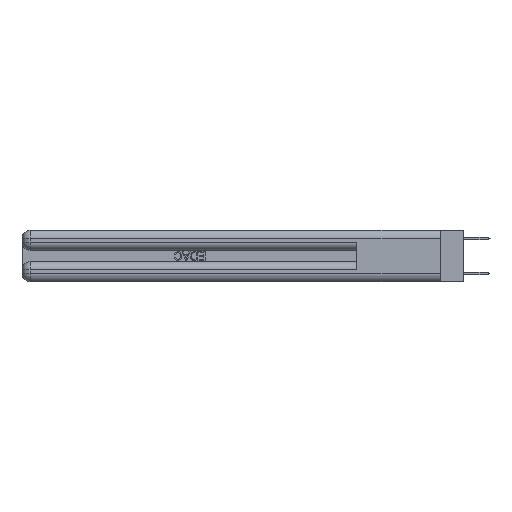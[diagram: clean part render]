
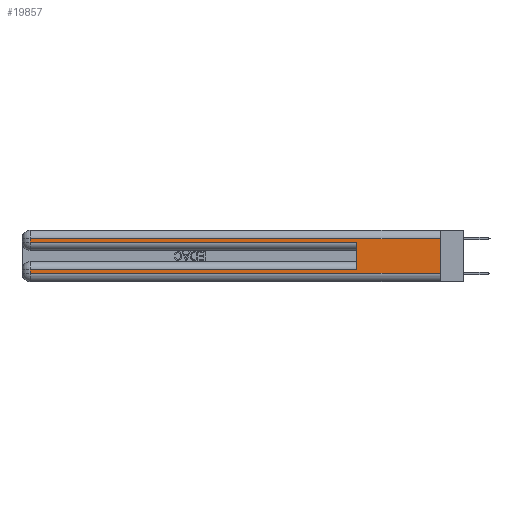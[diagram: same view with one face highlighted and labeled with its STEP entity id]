
A CAD part, left-side view. The second image highlights one B-rep face of the part: STEP entity #19857.
In plain terms, the highlighted planar face has unit normal (-1, 0, 0).
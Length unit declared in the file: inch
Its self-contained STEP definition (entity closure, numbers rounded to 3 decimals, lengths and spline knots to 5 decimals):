
#823 = ORIENTED_EDGE ( 'NONE', *, *, #7670, .T. ) ;
#1004 = CARTESIAN_POINT ( 'NONE',  ( 0., 2.94, 0.085 ) ) ;
#1013 = VECTOR ( 'NONE', #11278, 39.37008 ) ;
#1174 = CARTESIAN_POINT ( 'NONE',  ( 0., 2.94, 0.06 ) ) ;
#1431 = CARTESIAN_POINT ( 'NONE',  ( 0., 0., 0.085 ) ) ;
#1805 = LINE ( 'NONE', #6803, #30430 ) ;
#3520 = LINE ( 'NONE', #14603, #1013 ) ;
#3938 = DIRECTION ( 'NONE',  ( 0., -1., 0. ) ) ;
#4311 = ORIENTED_EDGE ( 'NONE', *, *, #22354, .T. ) ;
#4342 = LINE ( 'NONE', #21496, #29315 ) ;
#4529 = DIRECTION ( 'NONE',  ( 0., 1., 0. ) ) ;
#4663 = ORIENTED_EDGE ( 'NONE', *, *, #34394, .T. ) ;
#5802 = CARTESIAN_POINT ( 'NONE',  ( 0., 0., 0.37 ) ) ;
#6803 = CARTESIAN_POINT ( 'NONE',  ( 0., 0.6, 0.145 ) ) ;
#7670 = EDGE_CURVE ( 'NONE', #19176, #29488, #26688, .T. ) ;
#7906 = CARTESIAN_POINT ( 'NONE',  ( 0., 2.94, 0.37 ) ) ;
#8914 = PLANE ( 'NONE',  #16601 ) ;
#9913 = DIRECTION ( 'NONE',  ( 0., 1., 0. ) ) ;
#10883 = EDGE_CURVE ( 'NONE', #29488, #16420, #21374, .T. ) ;
#11278 = DIRECTION ( 'NONE',  ( 0., 0., -1. ) ) ;
#11532 = ORIENTED_EDGE ( 'NONE', *, *, #10883, .T. ) ;
#11798 = CARTESIAN_POINT ( 'NONE',  ( 0., 0., 0.285 ) ) ;
#12027 = VECTOR ( 'NONE', #9913, 39.37008 ) ;
#12035 = FACE_OUTER_BOUND ( 'NONE', #16592, .T. ) ;
#12646 = CARTESIAN_POINT ( 'NONE',  ( 0., 0.6, 0.085 ) ) ;
#12661 = EDGE_CURVE ( 'NONE', #24762, #19109, #17163, .T. ) ;
#12777 = ORIENTED_EDGE ( 'NONE', *, *, #12661, .T. ) ;
#13450 = CARTESIAN_POINT ( 'NONE',  ( 0., 0.6, 0.285 ) ) ;
#14570 = VERTEX_POINT ( 'NONE', #26330 ) ;
#14603 = CARTESIAN_POINT ( 'NONE',  ( 0., 2.94, 0.37 ) ) ;
#14660 = LINE ( 'NONE', #5802, #36129 ) ;
#15009 = ORIENTED_EDGE ( 'NONE', *, *, #25832, .F. ) ;
#15217 = ORIENTED_EDGE ( 'NONE', *, *, #31675, .F. ) ;
#15833 = VECTOR ( 'NONE', #23235, 39.37008 ) ;
#16107 = CARTESIAN_POINT ( 'NONE',  ( 0., 2.94, 0.285 ) ) ;
#16420 = VERTEX_POINT ( 'NONE', #1174 ) ;
#16592 = EDGE_LOOP ( 'NONE', ( #15009, #27000, #4663, #12777, #15217, #823, #11532, #4311 ) ) ;
#16601 = AXIS2_PLACEMENT_3D ( 'NONE', #28462, #23291, #22932 ) ;
#17163 = LINE ( 'NONE', #11798, #15833 ) ;
#18611 = DIRECTION ( 'NONE',  ( 0., 0., -1. ) ) ;
#19109 = VERTEX_POINT ( 'NONE', #13450 ) ;
#19176 = VERTEX_POINT ( 'NONE', #12646 ) ;
#19495 = CARTESIAN_POINT ( 'NONE',  ( 0., 0., 0.06 ) ) ;
#19857 = ADVANCED_FACE ( 'NONE', ( #12035 ), #8914, .F. ) ;
#21374 = LINE ( 'NONE', #7906, #30457 ) ;
#21496 = CARTESIAN_POINT ( 'NONE',  ( 0., 0., 0.31 ) ) ;
#22354 = EDGE_CURVE ( 'NONE', #16420, #32633, #30741, .T. ) ;
#22595 = DIRECTION ( 'NONE',  ( 0., 0., -1. ) ) ;
#22932 = DIRECTION ( 'NONE',  ( 0., 0., -1. ) ) ;
#23235 = DIRECTION ( 'NONE',  ( 0., -1., 0. ) ) ;
#23291 = DIRECTION ( 'NONE',  ( 1., 0., 0. ) ) ;
#24309 = DIRECTION ( 'NONE',  ( 0., 0., 1. ) ) ;
#24762 = VERTEX_POINT ( 'NONE', #16107 ) ;
#25832 = EDGE_CURVE ( 'NONE', #14570, #32633, #14660, .T. ) ;
#25881 = CARTESIAN_POINT ( 'NONE',  ( 0., 0., 0.06 ) ) ;
#26330 = CARTESIAN_POINT ( 'NONE',  ( 0., 0., 0.31 ) ) ;
#26648 = VECTOR ( 'NONE', #3938, 39.37008 ) ;
#26688 = LINE ( 'NONE', #1431, #12027 ) ;
#27000 = ORIENTED_EDGE ( 'NONE', *, *, #35054, .T. ) ;
#27485 = CARTESIAN_POINT ( 'NONE',  ( 0., 2.94, 0.31 ) ) ;
#28462 = CARTESIAN_POINT ( 'NONE',  ( 0., 0., 0.37 ) ) ;
#29315 = VECTOR ( 'NONE', #4529, 39.37008 ) ;
#29488 = VERTEX_POINT ( 'NONE', #1004 ) ;
#30430 = VECTOR ( 'NONE', #24309, 39.37008 ) ;
#30457 = VECTOR ( 'NONE', #18611, 39.37008 ) ;
#30741 = LINE ( 'NONE', #19495, #26648 ) ;
#31675 = EDGE_CURVE ( 'NONE', #19176, #19109, #1805, .T. ) ;
#32633 = VERTEX_POINT ( 'NONE', #25881 ) ;
#34394 = EDGE_CURVE ( 'NONE', #34832, #24762, #3520, .T. ) ;
#34832 = VERTEX_POINT ( 'NONE', #27485 ) ;
#35054 = EDGE_CURVE ( 'NONE', #14570, #34832, #4342, .T. ) ;
#36129 = VECTOR ( 'NONE', #22595, 39.37008 ) ;
